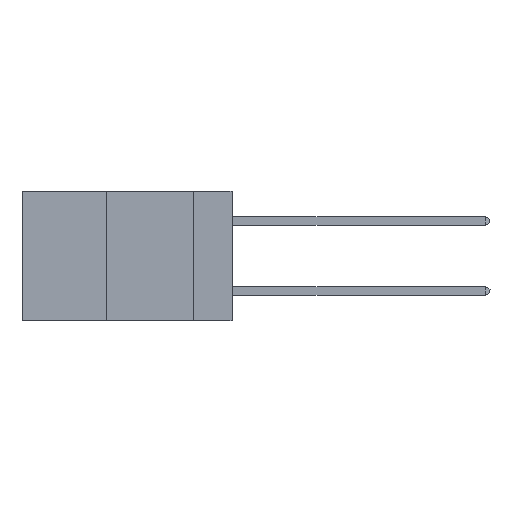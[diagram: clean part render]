
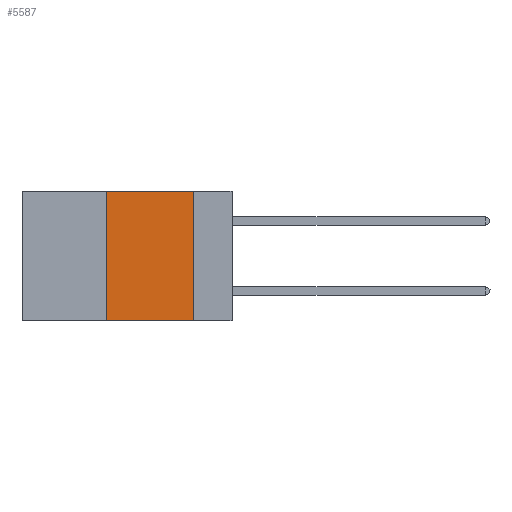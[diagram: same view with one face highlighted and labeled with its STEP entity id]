
A CAD part, left-side view. The second image highlights one B-rep face of the part: STEP entity #5587.
In plain terms, the highlighted planar face has unit normal (-1, 0, 0).
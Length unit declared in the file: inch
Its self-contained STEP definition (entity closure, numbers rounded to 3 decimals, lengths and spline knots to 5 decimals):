
#672 = EDGE_CURVE ( 'NONE', #721, #3037, #3884, .T. ) ;
#701 = CARTESIAN_POINT ( 'NONE',  ( 0., 0.36, 0. ) ) ;
#721 = VERTEX_POINT ( 'NONE', #805 ) ;
#805 = CARTESIAN_POINT ( 'NONE',  ( 0., 0.36, -0.37 ) ) ;
#1160 = DIRECTION ( 'NONE',  ( 0., 0., -1. ) ) ;
#1195 = PLANE ( 'NONE',  #2438 ) ;
#2011 = VECTOR ( 'NONE', #7699, 39.37008 ) ;
#2050 = CARTESIAN_POINT ( 'NONE',  ( 0., 0.11, 0. ) ) ;
#2102 = VERTEX_POINT ( 'NONE', #8005 ) ;
#2438 = AXIS2_PLACEMENT_3D ( 'NONE', #10006, #6004, #1160 ) ;
#2548 = DIRECTION ( 'NONE',  ( 0., -1., 0. ) ) ;
#2743 = ORIENTED_EDGE ( 'NONE', *, *, #672, .T. ) ;
#3037 = VERTEX_POINT ( 'NONE', #9975 ) ;
#3421 = VECTOR ( 'NONE', #7694, 39.37008 ) ;
#3499 = EDGE_LOOP ( 'NONE', ( #8990, #7211, #7350, #2743 ) ) ;
#3884 = LINE ( 'NONE', #8888, #8014 ) ;
#4618 = EDGE_CURVE ( 'NONE', #9160, #3037, #6214, .T. ) ;
#5189 = EDGE_CURVE ( 'NONE', #721, #2102, #9412, .T. ) ;
#5441 = DIRECTION ( 'NONE',  ( 0., 0., 1. ) ) ;
#5587 = ADVANCED_FACE ( 'NONE', ( #8659 ), #1195, .F. ) ;
#5940 = CARTESIAN_POINT ( 'NONE',  ( 0., 0.11, 0. ) ) ;
#6004 = DIRECTION ( 'NONE',  ( 1., 0., 0. ) ) ;
#6214 = LINE ( 'NONE', #2050, #3421 ) ;
#7211 = ORIENTED_EDGE ( 'NONE', *, *, #9652, .F. ) ;
#7350 = ORIENTED_EDGE ( 'NONE', *, *, #5189, .F. ) ;
#7371 = LINE ( 'NONE', #10145, #2011 ) ;
#7694 = DIRECTION ( 'NONE',  ( 0., 0., -1. ) ) ;
#7699 = DIRECTION ( 'NONE',  ( 0., -1., 0. ) ) ;
#8005 = CARTESIAN_POINT ( 'NONE',  ( 0., 0.36, 0. ) ) ;
#8014 = VECTOR ( 'NONE', #2548, 39.37008 ) ;
#8040 = VECTOR ( 'NONE', #5441, 39.37008 ) ;
#8659 = FACE_OUTER_BOUND ( 'NONE', #3499, .T. ) ;
#8888 = CARTESIAN_POINT ( 'NONE',  ( 0., 0.6, -0.37 ) ) ;
#8990 = ORIENTED_EDGE ( 'NONE', *, *, #4618, .F. ) ;
#9160 = VERTEX_POINT ( 'NONE', #5940 ) ;
#9412 = LINE ( 'NONE', #701, #8040 ) ;
#9652 = EDGE_CURVE ( 'NONE', #2102, #9160, #7371, .T. ) ;
#9975 = CARTESIAN_POINT ( 'NONE',  ( 0., 0.11, -0.37 ) ) ;
#10006 = CARTESIAN_POINT ( 'NONE',  ( 0., 0.6, 0. ) ) ;
#10145 = CARTESIAN_POINT ( 'NONE',  ( 0., 0.6, 0. ) ) ;
